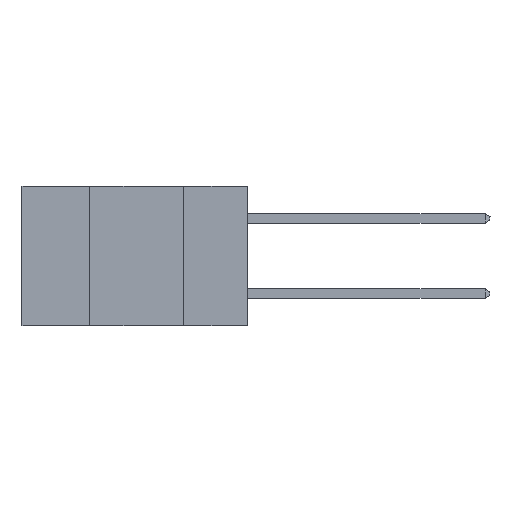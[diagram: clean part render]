
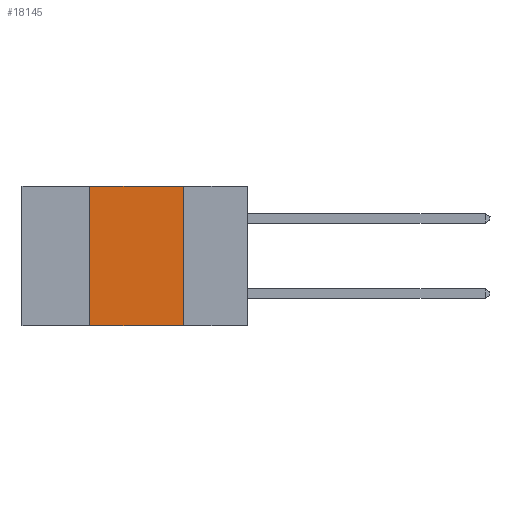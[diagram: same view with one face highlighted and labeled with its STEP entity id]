
A CAD part, left-side view. The second image highlights one B-rep face of the part: STEP entity #18145.
In plain terms, the highlighted planar face has unit normal (-1, 0, 0).
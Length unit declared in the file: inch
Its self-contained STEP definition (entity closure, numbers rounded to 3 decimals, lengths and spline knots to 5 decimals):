
#176 = VECTOR ( 'NONE', #11745, 39.37008 ) ;
#882 = AXIS2_PLACEMENT_3D ( 'NONE', #7388, #24427, #9364 ) ;
#2147 = CARTESIAN_POINT ( 'NONE',  ( 0., 0.17, 0. ) ) ;
#2488 = LINE ( 'NONE', #20254, #176 ) ;
#4223 = EDGE_CURVE ( 'NONE', #21786, #14088, #15839, .T. ) ;
#7388 = CARTESIAN_POINT ( 'NONE',  ( 0., 0.6, 0. ) ) ;
#7682 = DIRECTION ( 'NONE',  ( 0., -1., 0. ) ) ;
#7864 = EDGE_CURVE ( 'NONE', #13873, #14088, #21619, .T. ) ;
#9135 = ORIENTED_EDGE ( 'NONE', *, *, #4223, .T. ) ;
#9364 = DIRECTION ( 'NONE',  ( 0., 0., -1. ) ) ;
#9922 = CARTESIAN_POINT ( 'NONE',  ( 0., 0.42, 0. ) ) ;
#11745 = DIRECTION ( 'NONE',  ( 0., 0., 1. ) ) ;
#12586 = VECTOR ( 'NONE', #16672, 39.37008 ) ;
#13068 = VERTEX_POINT ( 'NONE', #9922 ) ;
#13473 = EDGE_CURVE ( 'NONE', #13068, #13873, #23985, .T. ) ;
#13873 = VERTEX_POINT ( 'NONE', #2147 ) ;
#14042 = EDGE_LOOP ( 'NONE', ( #16014, #16117, #16587, #9135 ) ) ;
#14088 = VERTEX_POINT ( 'NONE', #26527 ) ;
#15683 = PLANE ( 'NONE',  #882 ) ;
#15839 = LINE ( 'NONE', #24786, #21544 ) ;
#15920 = VECTOR ( 'NONE', #7682, 39.37008 ) ;
#16014 = ORIENTED_EDGE ( 'NONE', *, *, #7864, .F. ) ;
#16117 = ORIENTED_EDGE ( 'NONE', *, *, #13473, .F. ) ;
#16153 = DIRECTION ( 'NONE',  ( 0., -1., 0. ) ) ;
#16587 = ORIENTED_EDGE ( 'NONE', *, *, #25801, .F. ) ;
#16672 = DIRECTION ( 'NONE',  ( 0., 0., -1. ) ) ;
#18145 = ADVANCED_FACE ( 'NONE', ( #23553 ), #15683, .F. ) ;
#20254 = CARTESIAN_POINT ( 'NONE',  ( 0., 0.42, 0. ) ) ;
#20486 = CARTESIAN_POINT ( 'NONE',  ( 0., 0.6, 0. ) ) ;
#21544 = VECTOR ( 'NONE', #16153, 39.37008 ) ;
#21619 = LINE ( 'NONE', #27473, #12586 ) ;
#21786 = VERTEX_POINT ( 'NONE', #24638 ) ;
#23553 = FACE_OUTER_BOUND ( 'NONE', #14042, .T. ) ;
#23985 = LINE ( 'NONE', #20486, #15920 ) ;
#24427 = DIRECTION ( 'NONE',  ( 1., 0., 0. ) ) ;
#24638 = CARTESIAN_POINT ( 'NONE',  ( 0., 0.42, -0.37 ) ) ;
#24786 = CARTESIAN_POINT ( 'NONE',  ( 0., 0.6, -0.37 ) ) ;
#25801 = EDGE_CURVE ( 'NONE', #21786, #13068, #2488, .T. ) ;
#26527 = CARTESIAN_POINT ( 'NONE',  ( 0., 0.17, -0.37 ) ) ;
#27473 = CARTESIAN_POINT ( 'NONE',  ( 0., 0.17, 0. ) ) ;
